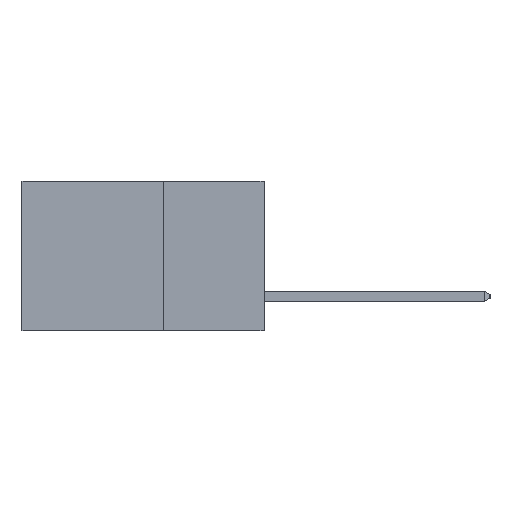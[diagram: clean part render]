
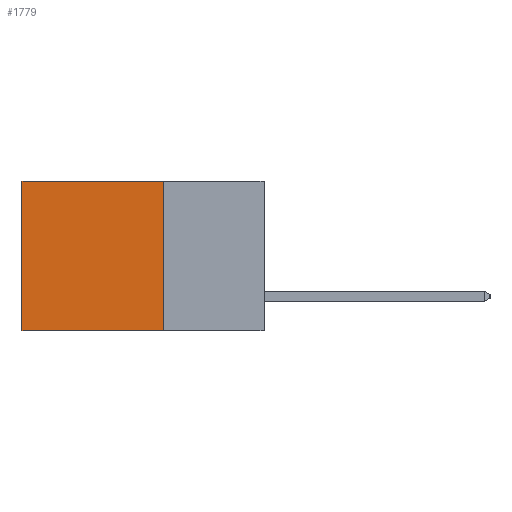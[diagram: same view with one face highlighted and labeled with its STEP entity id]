
A CAD part, left-side view. The second image highlights one B-rep face of the part: STEP entity #1779.
In plain terms, the highlighted planar face has unit normal (-1, 0, 0).
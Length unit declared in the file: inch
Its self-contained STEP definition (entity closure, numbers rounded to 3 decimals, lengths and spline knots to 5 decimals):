
#121 = LINE ( 'NONE', #10252, #10023 ) ;
#305 = CARTESIAN_POINT ( 'NONE',  ( 0.2615, 0.6, -0.37 ) ) ;
#449 = EDGE_CURVE ( 'NONE', #10809, #1535, #121, .T. ) ;
#652 = VERTEX_POINT ( 'NONE', #11264 ) ;
#1096 = VERTEX_POINT ( 'NONE', #305 ) ;
#1281 = CARTESIAN_POINT ( 'NONE',  ( 0.2615, 0.25, -0.37 ) ) ;
#1535 = VERTEX_POINT ( 'NONE', #11962 ) ;
#1779 = ADVANCED_FACE ( 'NONE', ( #11654 ), #1802, .F. ) ;
#1802 = PLANE ( 'NONE',  #14937 ) ;
#1816 = CARTESIAN_POINT ( 'NONE',  ( 0.2615, 0.6, -0.37 ) ) ;
#2162 = DIRECTION ( 'NONE',  ( 0., 0., -1. ) ) ;
#2983 = VECTOR ( 'NONE', #4412, 39.37008 ) ;
#3691 = EDGE_CURVE ( 'NONE', #10809, #652, #6781, .T. ) ;
#4412 = DIRECTION ( 'NONE',  ( 0., 1., 0. ) ) ;
#5004 = ORIENTED_EDGE ( 'NONE', *, *, #5540, .T. ) ;
#5178 = EDGE_CURVE ( 'NONE', #1535, #1096, #6420, .T. ) ;
#5398 = CARTESIAN_POINT ( 'NONE',  ( 0.2615, 0.25, -0.37 ) ) ;
#5540 = EDGE_CURVE ( 'NONE', #652, #1096, #7564, .T. ) ;
#5865 = ORIENTED_EDGE ( 'NONE', *, *, #5178, .F. ) ;
#6002 = ORIENTED_EDGE ( 'NONE', *, *, #449, .F. ) ;
#6420 = LINE ( 'NONE', #5398, #2983 ) ;
#6454 = DIRECTION ( 'NONE',  ( 1., 0., 0. ) ) ;
#6746 = ORIENTED_EDGE ( 'NONE', *, *, #3691, .T. ) ;
#6781 = LINE ( 'NONE', #8587, #10482 ) ;
#7233 = DIRECTION ( 'NONE',  ( 0., 0., -1. ) ) ;
#7564 = LINE ( 'NONE', #1816, #12908 ) ;
#8484 = DIRECTION ( 'NONE',  ( 0., 1., 0. ) ) ;
#8587 = CARTESIAN_POINT ( 'NONE',  ( 0.2615, 0.25, 0. ) ) ;
#10023 = VECTOR ( 'NONE', #7233, 39.37008 ) ;
#10252 = CARTESIAN_POINT ( 'NONE',  ( 0.2615, 0.25, -0.37 ) ) ;
#10482 = VECTOR ( 'NONE', #8484, 39.37008 ) ;
#10648 = DIRECTION ( 'NONE',  ( 0., 0., -1. ) ) ;
#10809 = VERTEX_POINT ( 'NONE', #11663 ) ;
#11264 = CARTESIAN_POINT ( 'NONE',  ( 0.2615, 0.6, 0. ) ) ;
#11654 = FACE_OUTER_BOUND ( 'NONE', #13750, .T. ) ;
#11663 = CARTESIAN_POINT ( 'NONE',  ( 0.2615, 0.25, 0. ) ) ;
#11962 = CARTESIAN_POINT ( 'NONE',  ( 0.2615, 0.25, -0.37 ) ) ;
#12908 = VECTOR ( 'NONE', #2162, 39.37008 ) ;
#13750 = EDGE_LOOP ( 'NONE', ( #5004, #5865, #6002, #6746 ) ) ;
#14937 = AXIS2_PLACEMENT_3D ( 'NONE', #1281, #6454, #10648 ) ;
